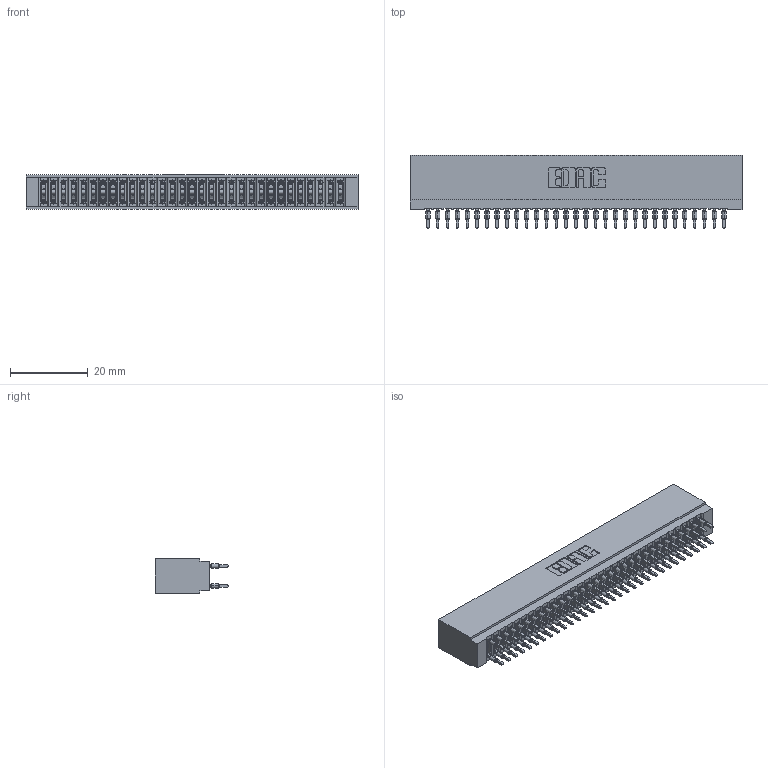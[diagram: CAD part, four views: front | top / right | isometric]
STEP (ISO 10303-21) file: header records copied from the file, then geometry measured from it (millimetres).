
FILE_DESCRIPTION (( 'STEP AP203' ), '1' );
FILE_NAME ('725-062-560-201.STEP', '2026-02-24T18:19:17', ( '' ), ( '' ), 'SwSTEP 2.0', 'SolidWorks 2023', '' );
FILE_SCHEMA (( 'CONFIG_CONTROL_DESIGN' ));
Length unit declared in the file: millimetre
Products named in the file (3): 725-062-560-201; 745-292-001_560; 725 Part_Insulator Option - 01
Assembly tree (63 placements, depth 2):
  725-062-560-201
    725 Part_Insulator Option - 01
    745-292-001_560  x62
Bounding box: 85.34 x 18.8 x 8.89 mm (x, y, z)
Volume: 7052.3 mm3; surface area: 15637.7 mm2
Topology: 63 solids, 63 shells, 6202 faces, 16963 edges, 10770 vertices
Faces by surface type: plane 3217, cylinder 1373, bspline 1240, torus 372
Entity records: 53978 total; most frequent: CARTESIAN_POINT 9869, ORIENTED_EDGE 9282, DIRECTION 8125, EDGE_CURVE 4641, VECTOR 4265, LINE 4265, VERTEX_POINT 2962, AXIS2_PLACEMENT_3D 1930
